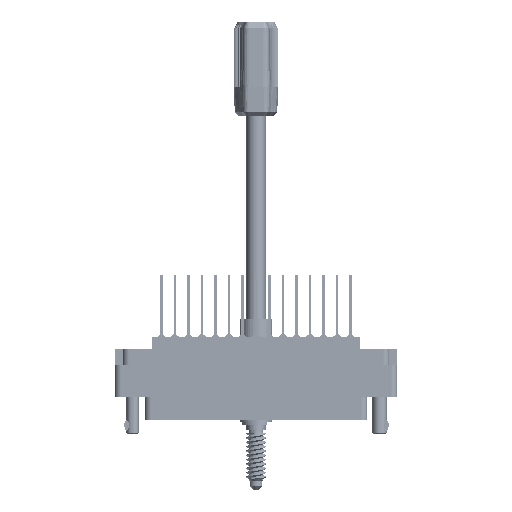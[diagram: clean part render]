
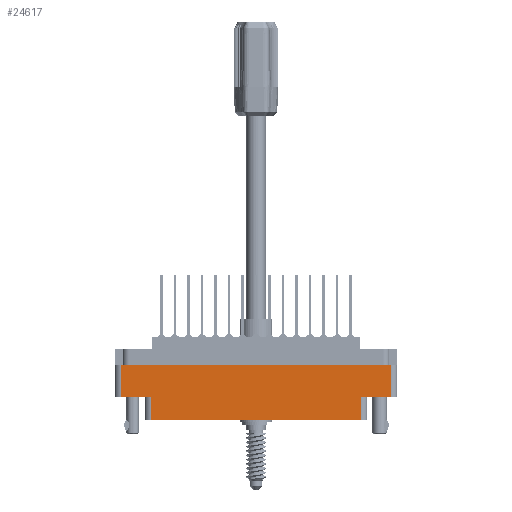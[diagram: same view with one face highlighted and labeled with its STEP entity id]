
A CAD part, front view. The second image highlights one B-rep face of the part: STEP entity #24617.
In plain terms, the highlighted planar face has unit normal (0, -1, 0).
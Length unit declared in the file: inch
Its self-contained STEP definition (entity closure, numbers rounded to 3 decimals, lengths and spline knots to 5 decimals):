
#381 = EDGE_CURVE ( 'NONE', #39357, #17054, #86699, .T. ) ;
#635 = VECTOR ( 'NONE', #36357, 39.37008 ) ;
#1441 = CARTESIAN_POINT ( 'NONE',  ( 1.006, -0.617, -0.578 ) ) ;
#3653 = VERTEX_POINT ( 'NONE', #7592 ) ;
#4023 = DIRECTION ( 'NONE',  ( 1., 0., 0. ) ) ;
#5763 = VERTEX_POINT ( 'NONE', #89738 ) ;
#6081 = DIRECTION ( 'NONE',  ( 1., 0., 0. ) ) ;
#6398 = CARTESIAN_POINT ( 'NONE',  ( 0., -0.617, -0.578 ) ) ;
#7592 = CARTESIAN_POINT ( 'NONE',  ( -1.006, -0.617, -0.578 ) ) ;
#7753 = EDGE_CURVE ( 'NONE', #91356, #39357, #42564, .T. ) ;
#9705 = PLANE ( 'NONE',  #80266 ) ;
#10333 = ORIENTED_EDGE ( 'NONE', *, *, #7753, .T. ) ;
#10595 = VECTOR ( 'NONE', #18895, 39.37008 ) ;
#11043 = CARTESIAN_POINT ( 'NONE',  ( 1.297, -0.617, -0.578 ) ) ;
#11741 = EDGE_CURVE ( 'NONE', #44913, #5763, #65814, .T. ) ;
#14058 = CARTESIAN_POINT ( 'NONE',  ( 1.297, -0.617, -0.798 ) ) ;
#15499 = VECTOR ( 'NONE', #6081, 39.37008 ) ;
#17054 = VERTEX_POINT ( 'NONE', #71037 ) ;
#17624 = EDGE_CURVE ( 'NONE', #3653, #91356, #52640, .T. ) ;
#18895 = DIRECTION ( 'NONE',  ( 0., 0., -1. ) ) ;
#20444 = CARTESIAN_POINT ( 'NONE',  ( -1.006, -0.617, -0.798 ) ) ;
#22582 = ORIENTED_EDGE ( 'NONE', *, *, #51237, .T. ) ;
#22874 = CARTESIAN_POINT ( 'NONE',  ( 1.006, -0.617, -0.798 ) ) ;
#24617 = ADVANCED_FACE ( 'NONE', ( #29835 ), #9705, .T. ) ;
#27565 = VECTOR ( 'NONE', #36507, 39.37008 ) ;
#28589 = CARTESIAN_POINT ( 'NONE',  ( -1.006, -0.617, -0.798 ) ) ;
#29835 = FACE_OUTER_BOUND ( 'NONE', #87943, .T. ) ;
#31322 = DIRECTION ( 'NONE',  ( 1., 0., 0. ) ) ;
#34375 = CARTESIAN_POINT ( 'NONE',  ( -1.297, -0.617, -0.274 ) ) ;
#35609 = CARTESIAN_POINT ( 'NONE',  ( -1.297, -0.617, -0.578 ) ) ;
#36357 = DIRECTION ( 'NONE',  ( 0., 0., 1. ) ) ;
#36507 = DIRECTION ( 'NONE',  ( 0., 0., -1. ) ) ;
#37759 = DIRECTION ( 'NONE',  ( 0., -1., 0. ) ) ;
#38956 = ORIENTED_EDGE ( 'NONE', *, *, #41864, .T. ) ;
#39068 = DIRECTION ( 'NONE',  ( 0., 0., 1. ) ) ;
#39357 = VERTEX_POINT ( 'NONE', #22874 ) ;
#40505 = LINE ( 'NONE', #14058, #635 ) ;
#41864 = EDGE_CURVE ( 'NONE', #44913, #52071, #87033, .T. ) ;
#42564 = LINE ( 'NONE', #68128, #80284 ) ;
#44913 = VERTEX_POINT ( 'NONE', #34375 ) ;
#48887 = CARTESIAN_POINT ( 'NONE',  ( 0., -0.617, -0.578 ) ) ;
#51237 = EDGE_CURVE ( 'NONE', #90713, #5763, #40505, .T. ) ;
#52071 = VERTEX_POINT ( 'NONE', #35609 ) ;
#52487 = EDGE_CURVE ( 'NONE', #90713, #17054, #55802, .T. ) ;
#52640 = LINE ( 'NONE', #28589, #27565 ) ;
#55583 = CARTESIAN_POINT ( 'NONE',  ( -1.297, -0.617, -0.798 ) ) ;
#55802 = LINE ( 'NONE', #6398, #57004 ) ;
#56194 = ORIENTED_EDGE ( 'NONE', *, *, #17624, .T. ) ;
#57004 = VECTOR ( 'NONE', #57438, 39.37008 ) ;
#57438 = DIRECTION ( 'NONE',  ( -1., 0., 0. ) ) ;
#63701 = ORIENTED_EDGE ( 'NONE', *, *, #71146, .T. ) ;
#65814 = LINE ( 'NONE', #67948, #91052 ) ;
#66796 = DIRECTION ( 'NONE',  ( 0., 0., -1. ) ) ;
#67948 = CARTESIAN_POINT ( 'NONE',  ( 0., -0.617, -0.274 ) ) ;
#68128 = CARTESIAN_POINT ( 'NONE',  ( -1.359, -0.617, -0.798 ) ) ;
#68602 = ORIENTED_EDGE ( 'NONE', *, *, #381, .T. ) ;
#71037 = CARTESIAN_POINT ( 'NONE',  ( 1.006, -0.617, -0.578 ) ) ;
#71146 = EDGE_CURVE ( 'NONE', #52071, #3653, #73692, .T. ) ;
#73692 = LINE ( 'NONE', #48887, #15499 ) ;
#75367 = ORIENTED_EDGE ( 'NONE', *, *, #11741, .F. ) ;
#80266 = AXIS2_PLACEMENT_3D ( 'NONE', #89172, #37759, #66796 ) ;
#80284 = VECTOR ( 'NONE', #4023, 39.37008 ) ;
#84034 = ORIENTED_EDGE ( 'NONE', *, *, #52487, .F. ) ;
#86699 = LINE ( 'NONE', #1441, #89005 ) ;
#87033 = LINE ( 'NONE', #55583, #10595 ) ;
#87943 = EDGE_LOOP ( 'NONE', ( #63701, #56194, #10333, #68602, #84034, #22582, #75367, #38956 ) ) ;
#89005 = VECTOR ( 'NONE', #39068, 39.37008 ) ;
#89172 = CARTESIAN_POINT ( 'NONE',  ( -1.359, -0.617, -0.798 ) ) ;
#89738 = CARTESIAN_POINT ( 'NONE',  ( 1.297, -0.617, -0.274 ) ) ;
#90713 = VERTEX_POINT ( 'NONE', #11043 ) ;
#91052 = VECTOR ( 'NONE', #31322, 39.37008 ) ;
#91356 = VERTEX_POINT ( 'NONE', #20444 ) ;
